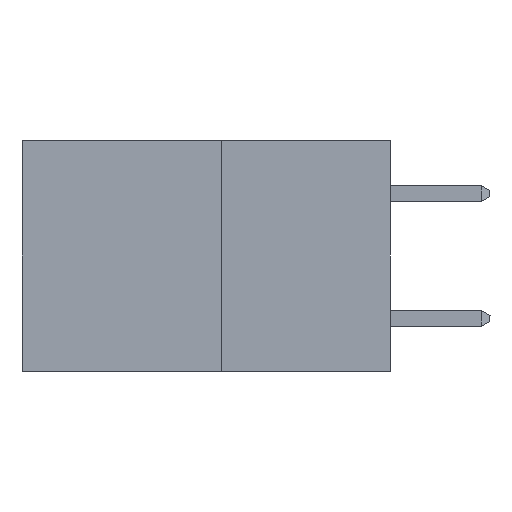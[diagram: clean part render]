
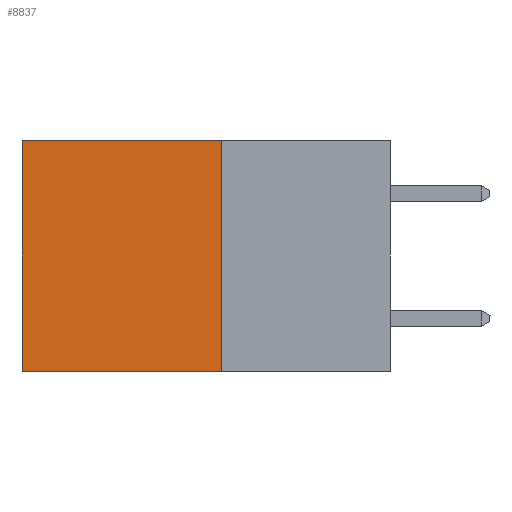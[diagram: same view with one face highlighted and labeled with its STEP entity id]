
A CAD part, left-side view. The second image highlights one B-rep face of the part: STEP entity #8837.
In plain terms, the highlighted planar face has unit normal (-1, 0, 0).
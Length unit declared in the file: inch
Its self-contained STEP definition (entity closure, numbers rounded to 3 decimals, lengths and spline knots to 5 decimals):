
#174 = PLANE ( 'NONE',  #9792 ) ;
#360 = VECTOR ( 'NONE', #389, 39.37008 ) ;
#389 = DIRECTION ( 'NONE',  ( 0., 1., 0. ) ) ;
#586 = VERTEX_POINT ( 'NONE', #9662 ) ;
#788 = FACE_OUTER_BOUND ( 'NONE', #3556, .T. ) ;
#905 = CARTESIAN_POINT ( 'NONE',  ( 0.277, 0.27, 0. ) ) ;
#913 = DIRECTION ( 'NONE',  ( 0., 0., -1. ) ) ;
#1454 = ORIENTED_EDGE ( 'NONE', *, *, #8356, .F. ) ;
#1526 = CARTESIAN_POINT ( 'NONE',  ( 0.277, 0.59, 0. ) ) ;
#1562 = DIRECTION ( 'NONE',  ( 0., 0., -1. ) ) ;
#2668 = CARTESIAN_POINT ( 'NONE',  ( 0.277, 0.27, 0. ) ) ;
#2824 = DIRECTION ( 'NONE',  ( 0., 1., 0. ) ) ;
#2897 = VECTOR ( 'NONE', #913, 39.37008 ) ;
#3024 = LINE ( 'NONE', #6658, #9506 ) ;
#3077 = DIRECTION ( 'NONE',  ( 0., 0., -1. ) ) ;
#3156 = LINE ( 'NONE', #10938, #2897 ) ;
#3275 = LINE ( 'NONE', #905, #7167 ) ;
#3417 = VERTEX_POINT ( 'NONE', #1526 ) ;
#3481 = VERTEX_POINT ( 'NONE', #2668 ) ;
#3556 = EDGE_LOOP ( 'NONE', ( #9712, #9632, #1454, #9859 ) ) ;
#3894 = EDGE_CURVE ( 'NONE', #3481, #3417, #3275, .T. ) ;
#3934 = VERTEX_POINT ( 'NONE', #9343 ) ;
#4661 = CARTESIAN_POINT ( 'NONE',  ( 0.277, 0.27, -0.37 ) ) ;
#4929 = CARTESIAN_POINT ( 'NONE',  ( 0.277, 0.27, -0.37 ) ) ;
#5211 = LINE ( 'NONE', #4929, #360 ) ;
#6528 = EDGE_CURVE ( 'NONE', #3934, #586, #5211, .T. ) ;
#6658 = CARTESIAN_POINT ( 'NONE',  ( 0.277, 0.27, -0.37 ) ) ;
#7167 = VECTOR ( 'NONE', #2824, 39.37008 ) ;
#8010 = DIRECTION ( 'NONE',  ( 1., 0., 0. ) ) ;
#8356 = EDGE_CURVE ( 'NONE', #3481, #3934, #3024, .T. ) ;
#8637 = EDGE_CURVE ( 'NONE', #3417, #586, #3156, .T. ) ;
#8837 = ADVANCED_FACE ( 'NONE', ( #788 ), #174, .F. ) ;
#9343 = CARTESIAN_POINT ( 'NONE',  ( 0.277, 0.27, -0.37 ) ) ;
#9506 = VECTOR ( 'NONE', #1562, 39.37008 ) ;
#9632 = ORIENTED_EDGE ( 'NONE', *, *, #6528, .F. ) ;
#9662 = CARTESIAN_POINT ( 'NONE',  ( 0.277, 0.59, -0.37 ) ) ;
#9712 = ORIENTED_EDGE ( 'NONE', *, *, #8637, .T. ) ;
#9792 = AXIS2_PLACEMENT_3D ( 'NONE', #4661, #8010, #3077 ) ;
#9859 = ORIENTED_EDGE ( 'NONE', *, *, #3894, .T. ) ;
#10938 = CARTESIAN_POINT ( 'NONE',  ( 0.277, 0.59, -0.37 ) ) ;
